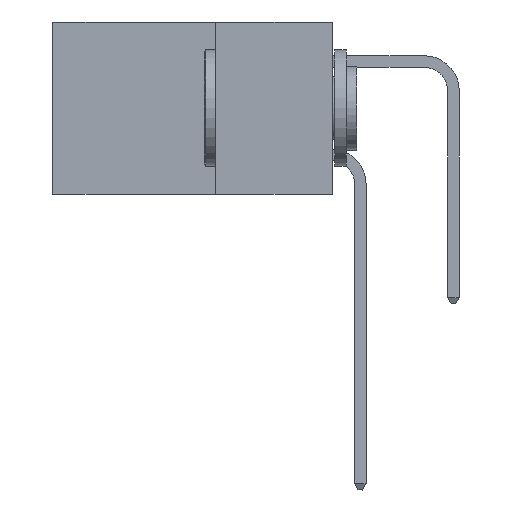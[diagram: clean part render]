
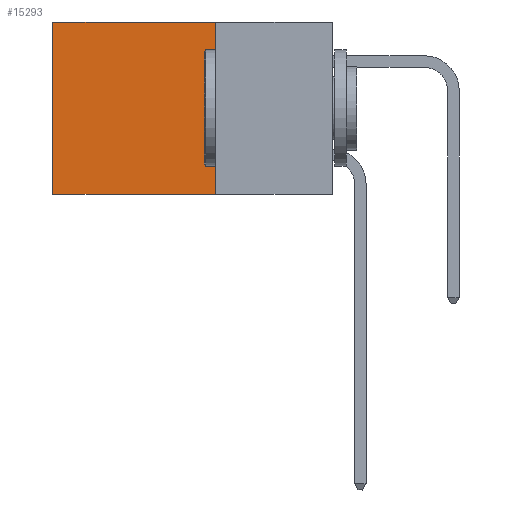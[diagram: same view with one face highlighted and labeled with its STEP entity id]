
A CAD part, left-side view. The second image highlights one B-rep face of the part: STEP entity #15293.
In plain terms, the highlighted planar face has unit normal (-1, 0, 0).
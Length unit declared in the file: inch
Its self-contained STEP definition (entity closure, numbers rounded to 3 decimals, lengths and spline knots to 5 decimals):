
#322 = DIRECTION ( 'NONE',  ( 0., 0., -1. ) ) ;
#1534 = VECTOR ( 'NONE', #322, 39.37008 ) ;
#2375 = VECTOR ( 'NONE', #13085, 39.37008 ) ;
#2607 = LINE ( 'NONE', #12559, #19993 ) ;
#3051 = ORIENTED_EDGE ( 'NONE', *, *, #8942, .T. ) ;
#5384 = LINE ( 'NONE', #14215, #1534 ) ;
#5575 = VERTEX_POINT ( 'NONE', #15627 ) ;
#5691 = DIRECTION ( 'NONE',  ( 0., 0., -1. ) ) ;
#5828 = CARTESIAN_POINT ( 'NONE',  ( 0.2615, 0.25, -0.37 ) ) ;
#6481 = EDGE_CURVE ( 'NONE', #18950, #13453, #5384, .T. ) ;
#6759 = DIRECTION ( 'NONE',  ( 0., 1., 0. ) ) ;
#7721 = EDGE_CURVE ( 'NONE', #13453, #11904, #17135, .T. ) ;
#7822 = DIRECTION ( 'NONE',  ( 0., 0., -1. ) ) ;
#8192 = CARTESIAN_POINT ( 'NONE',  ( 0.2615, 0.6, -0.37 ) ) ;
#8942 = EDGE_CURVE ( 'NONE', #18950, #5575, #9551, .T. ) ;
#9551 = LINE ( 'NONE', #13193, #2375 ) ;
#11160 = DIRECTION ( 'NONE',  ( 1., 0., 0. ) ) ;
#11676 = EDGE_LOOP ( 'NONE', ( #14849, #16283, #21305, #3051 ) ) ;
#11904 = VERTEX_POINT ( 'NONE', #8192 ) ;
#11974 = CARTESIAN_POINT ( 'NONE',  ( 0.2615, 0.25, -0.37 ) ) ;
#12559 = CARTESIAN_POINT ( 'NONE',  ( 0.2615, 0.6, -0.37 ) ) ;
#12983 = VECTOR ( 'NONE', #6759, 39.37008 ) ;
#13085 = DIRECTION ( 'NONE',  ( 0., 1., 0. ) ) ;
#13193 = CARTESIAN_POINT ( 'NONE',  ( 0.2615, 0.25, 0. ) ) ;
#13453 = VERTEX_POINT ( 'NONE', #18988 ) ;
#14215 = CARTESIAN_POINT ( 'NONE',  ( 0.2615, 0.25, -0.37 ) ) ;
#14221 = PLANE ( 'NONE',  #16875 ) ;
#14360 = EDGE_CURVE ( 'NONE', #5575, #11904, #2607, .T. ) ;
#14849 = ORIENTED_EDGE ( 'NONE', *, *, #14360, .T. ) ;
#15293 = ADVANCED_FACE ( 'NONE', ( #15771 ), #14221, .F. ) ;
#15569 = CARTESIAN_POINT ( 'NONE',  ( 0.2615, 0.25, 0. ) ) ;
#15627 = CARTESIAN_POINT ( 'NONE',  ( 0.2615, 0.6, 0. ) ) ;
#15771 = FACE_OUTER_BOUND ( 'NONE', #11676, .T. ) ;
#16283 = ORIENTED_EDGE ( 'NONE', *, *, #7721, .F. ) ;
#16875 = AXIS2_PLACEMENT_3D ( 'NONE', #5828, #11160, #7822 ) ;
#17135 = LINE ( 'NONE', #11974, #12983 ) ;
#18950 = VERTEX_POINT ( 'NONE', #15569 ) ;
#18988 = CARTESIAN_POINT ( 'NONE',  ( 0.2615, 0.25, -0.37 ) ) ;
#19993 = VECTOR ( 'NONE', #5691, 39.37008 ) ;
#21305 = ORIENTED_EDGE ( 'NONE', *, *, #6481, .F. ) ;
